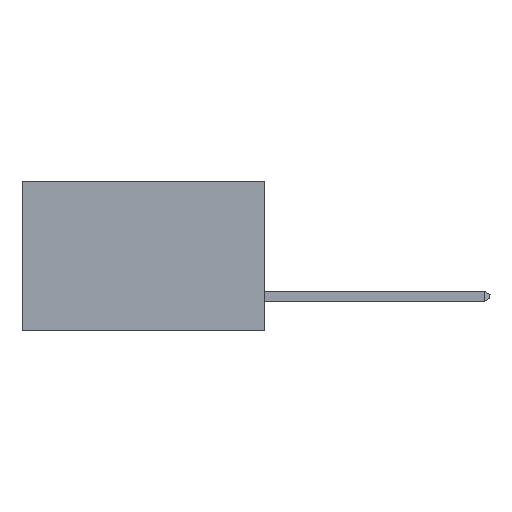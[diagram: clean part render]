
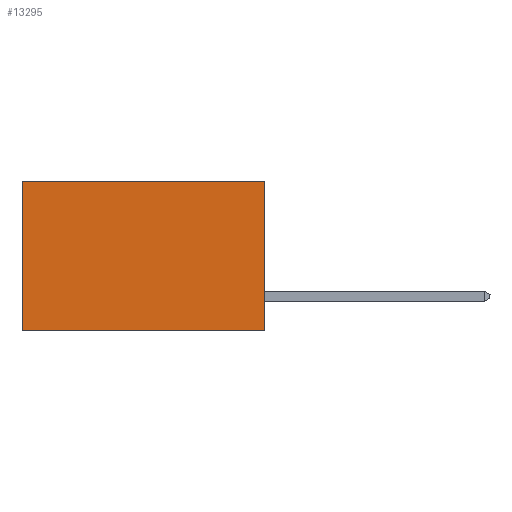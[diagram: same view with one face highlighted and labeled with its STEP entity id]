
A CAD part, left-side view. The second image highlights one B-rep face of the part: STEP entity #13295.
In plain terms, the highlighted planar face has unit normal (-1, 0, 0).
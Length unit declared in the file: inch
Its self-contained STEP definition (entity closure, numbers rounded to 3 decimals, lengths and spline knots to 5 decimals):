
#459 = DIRECTION ( 'NONE',  ( 0., 1., 0. ) ) ;
#798 = CARTESIAN_POINT ( 'NONE',  ( 0.298, 0., 0. ) ) ;
#2281 = CARTESIAN_POINT ( 'NONE',  ( 0.298, 0.6, 0. ) ) ;
#2410 = FACE_OUTER_BOUND ( 'NONE', #5452, .T. ) ;
#2512 = VECTOR ( 'NONE', #459, 39.37008 ) ;
#3146 = VERTEX_POINT ( 'NONE', #3702 ) ;
#3702 = CARTESIAN_POINT ( 'NONE',  ( 0.298, 0., -0.37 ) ) ;
#3787 = VERTEX_POINT ( 'NONE', #5481 ) ;
#5452 = EDGE_LOOP ( 'NONE', ( #12306, #18071, #19409, #11445 ) ) ;
#5481 = CARTESIAN_POINT ( 'NONE',  ( 0.298, 0.6, 0. ) ) ;
#5546 = CARTESIAN_POINT ( 'NONE',  ( 0.298, 0., 0. ) ) ;
#6249 = VERTEX_POINT ( 'NONE', #16529 ) ;
#6264 = VECTOR ( 'NONE', #15440, 39.37008 ) ;
#6970 = LINE ( 'NONE', #2281, #18642 ) ;
#7480 = EDGE_CURVE ( 'NONE', #3146, #6249, #18723, .T. ) ;
#8375 = VECTOR ( 'NONE', #16119, 39.37008 ) ;
#9311 = CARTESIAN_POINT ( 'NONE',  ( 0.298, 0., 0. ) ) ;
#11145 = DIRECTION ( 'NONE',  ( 1., 0., 0. ) ) ;
#11222 = LINE ( 'NONE', #5546, #8375 ) ;
#11402 = DIRECTION ( 'NONE',  ( 0., 0., -1. ) ) ;
#11445 = ORIENTED_EDGE ( 'NONE', *, *, #16079, .T. ) ;
#12306 = ORIENTED_EDGE ( 'NONE', *, *, #17402, .T. ) ;
#12978 = EDGE_CURVE ( 'NONE', #15672, #3146, #11222, .T. ) ;
#13295 = ADVANCED_FACE ( 'NONE', ( #2410 ), #22223, .F. ) ;
#15440 = DIRECTION ( 'NONE',  ( 0., 1., 0. ) ) ;
#15672 = VERTEX_POINT ( 'NONE', #21465 ) ;
#16079 = EDGE_CURVE ( 'NONE', #15672, #3787, #19725, .T. ) ;
#16119 = DIRECTION ( 'NONE',  ( 0., 0., -1. ) ) ;
#16529 = CARTESIAN_POINT ( 'NONE',  ( 0.298, 0.6, -0.37 ) ) ;
#16800 = CARTESIAN_POINT ( 'NONE',  ( 0.298, 0., -0.37 ) ) ;
#17402 = EDGE_CURVE ( 'NONE', #3787, #6249, #6970, .T. ) ;
#18071 = ORIENTED_EDGE ( 'NONE', *, *, #7480, .F. ) ;
#18642 = VECTOR ( 'NONE', #11402, 39.37008 ) ;
#18723 = LINE ( 'NONE', #16800, #2512 ) ;
#19409 = ORIENTED_EDGE ( 'NONE', *, *, #12978, .F. ) ;
#19725 = LINE ( 'NONE', #798, #6264 ) ;
#21240 = AXIS2_PLACEMENT_3D ( 'NONE', #9311, #11145, #22144 ) ;
#21465 = CARTESIAN_POINT ( 'NONE',  ( 0.298, 0., 0. ) ) ;
#22144 = DIRECTION ( 'NONE',  ( 0., 0., -1. ) ) ;
#22223 = PLANE ( 'NONE',  #21240 ) ;
